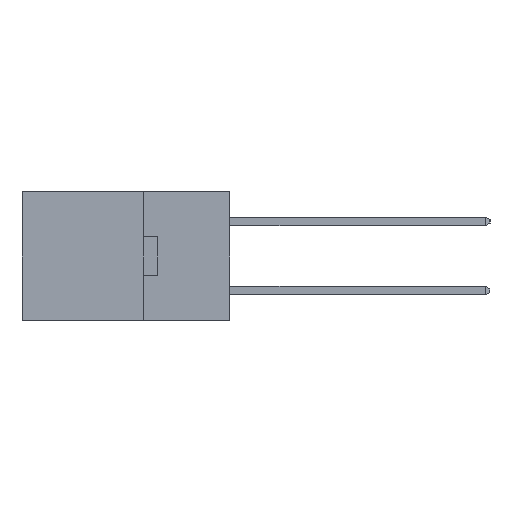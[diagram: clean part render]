
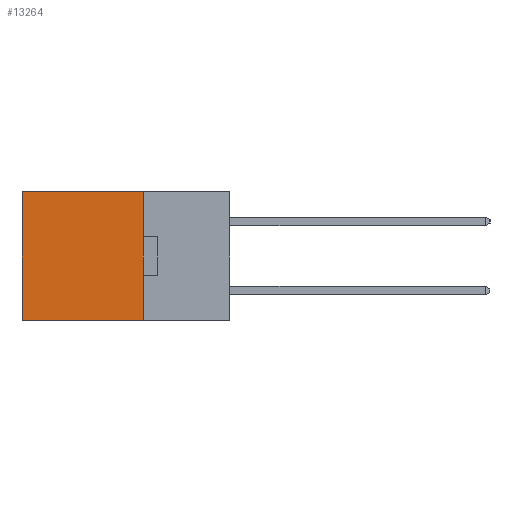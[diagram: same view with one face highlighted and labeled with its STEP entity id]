
A CAD part, left-side view. The second image highlights one B-rep face of the part: STEP entity #13264.
In plain terms, the highlighted planar face has unit normal (-1, 0, 0).
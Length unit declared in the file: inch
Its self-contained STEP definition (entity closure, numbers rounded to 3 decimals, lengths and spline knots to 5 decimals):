
#356 = VECTOR ( 'NONE', #11973, 39.37008 ) ;
#1400 = LINE ( 'NONE', #9774, #356 ) ;
#2194 = EDGE_LOOP ( 'NONE', ( #5039, #7175, #24495, #19191 ) ) ;
#2593 = CARTESIAN_POINT ( 'NONE',  ( 0.2615, 0.25, 0. ) ) ;
#4286 = VERTEX_POINT ( 'NONE', #7077 ) ;
#4953 = EDGE_CURVE ( 'NONE', #24087, #19946, #12008, .T. ) ;
#4981 = CARTESIAN_POINT ( 'NONE',  ( 0.2615, 0.6, -0.37 ) ) ;
#5039 = ORIENTED_EDGE ( 'NONE', *, *, #4953, .T. ) ;
#5845 = EDGE_CURVE ( 'NONE', #13460, #24087, #1400, .T. ) ;
#6413 = VECTOR ( 'NONE', #15824, 39.37008 ) ;
#7077 = CARTESIAN_POINT ( 'NONE',  ( 0.2615, 0.25, -0.37 ) ) ;
#7137 = VECTOR ( 'NONE', #27258, 39.37008 ) ;
#7175 = ORIENTED_EDGE ( 'NONE', *, *, #9436, .F. ) ;
#8948 = EDGE_CURVE ( 'NONE', #13460, #4286, #12959, .T. ) ;
#8976 = FACE_OUTER_BOUND ( 'NONE', #2194, .T. ) ;
#9436 = EDGE_CURVE ( 'NONE', #4286, #19946, #23745, .T. ) ;
#9774 = CARTESIAN_POINT ( 'NONE',  ( 0.2615, 0.25, 0. ) ) ;
#9980 = CARTESIAN_POINT ( 'NONE',  ( 0.2615, 0.25, -0.37 ) ) ;
#10729 = PLANE ( 'NONE',  #20653 ) ;
#11302 = VECTOR ( 'NONE', #20125, 39.37008 ) ;
#11418 = CARTESIAN_POINT ( 'NONE',  ( 0.2615, 0.25, -0.37 ) ) ;
#11973 = DIRECTION ( 'NONE',  ( 0., 1., 0. ) ) ;
#12008 = LINE ( 'NONE', #15738, #11302 ) ;
#12959 = LINE ( 'NONE', #9980, #7137 ) ;
#13044 = DIRECTION ( 'NONE',  ( 1., 0., 0. ) ) ;
#13264 = ADVANCED_FACE ( 'NONE', ( #8976 ), #10729, .F. ) ;
#13460 = VERTEX_POINT ( 'NONE', #2593 ) ;
#15738 = CARTESIAN_POINT ( 'NONE',  ( 0.2615, 0.6, -0.37 ) ) ;
#15824 = DIRECTION ( 'NONE',  ( 0., 1., 0. ) ) ;
#16875 = CARTESIAN_POINT ( 'NONE',  ( 0.2615, 0.6, 0. ) ) ;
#19191 = ORIENTED_EDGE ( 'NONE', *, *, #5845, .T. ) ;
#19946 = VERTEX_POINT ( 'NONE', #4981 ) ;
#20125 = DIRECTION ( 'NONE',  ( 0., 0., -1. ) ) ;
#20653 = AXIS2_PLACEMENT_3D ( 'NONE', #25936, #13044, #26890 ) ;
#23745 = LINE ( 'NONE', #11418, #6413 ) ;
#24087 = VERTEX_POINT ( 'NONE', #16875 ) ;
#24495 = ORIENTED_EDGE ( 'NONE', *, *, #8948, .F. ) ;
#25936 = CARTESIAN_POINT ( 'NONE',  ( 0.2615, 0.25, -0.37 ) ) ;
#26890 = DIRECTION ( 'NONE',  ( 0., 0., -1. ) ) ;
#27258 = DIRECTION ( 'NONE',  ( 0., 0., -1. ) ) ;
